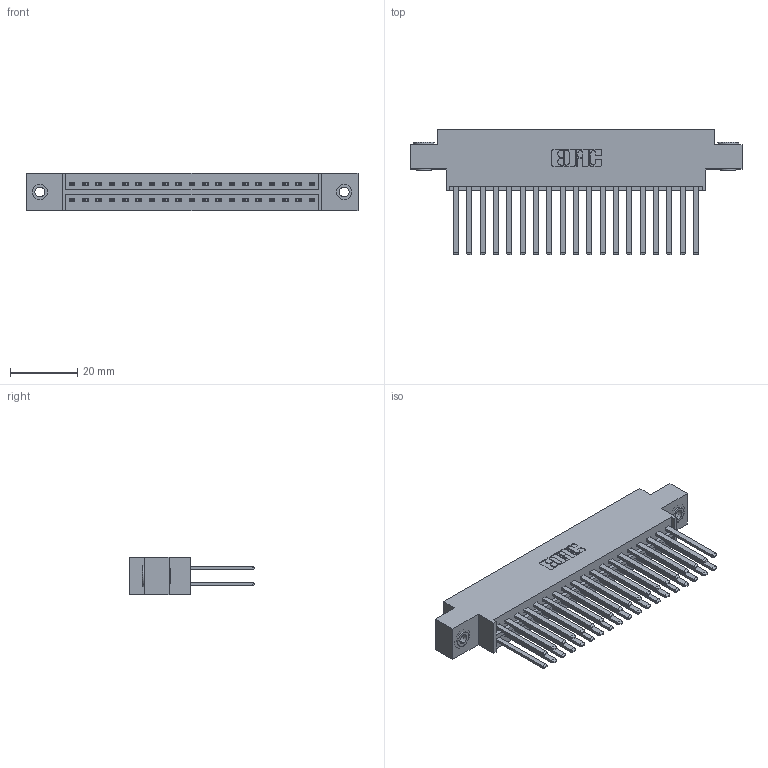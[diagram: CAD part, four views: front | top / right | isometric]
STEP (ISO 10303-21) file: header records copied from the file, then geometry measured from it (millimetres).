
FILE_DESCRIPTION (( 'STEP AP203' ), '1' );
FILE_NAME ('336-038-541-803.STEP', '2020-08-07T23:04:18', ( '' ), ( '' ), 'SwSTEP 2.0', 'SolidWorks 2020', '' );
FILE_SCHEMA (( 'CONFIG_CONTROL_DESIGN' ));
Length unit declared in the file: inch
Products named in the file (4): 336-290-001_336-290-541; 345-250-002_345-250-002-102; 336 Part_Offset - .156 Dia - TH; 336-038-541-803
Assembly tree (41 placements, depth 2):
  336-038-541-803
    336 Part_Offset - .156 Dia - TH
    336-290-001_336-290-541  x38
    345-250-002_345-250-002-102  x2
Bounding box: 98.68 x 37.34 x 11.1 mm (x, y, z)
Volume: 14502.3 mm3; surface area: 18366.9 mm2
Topology: 41 solids, 41 shells, 1752 faces, 5225 edges, 3454 vertices
Faces by surface type: plane 1072, cylinder 672, cone 8
Entity records: 18207 total; most frequent: CARTESIAN_POINT 3144, ORIENTED_EDGE 2974, DIRECTION 2653, EDGE_CURVE 1487, VECTOR 1331, LINE 1331, VERTEX_POINT 988, AXIS2_PLACEMENT_3D 661
